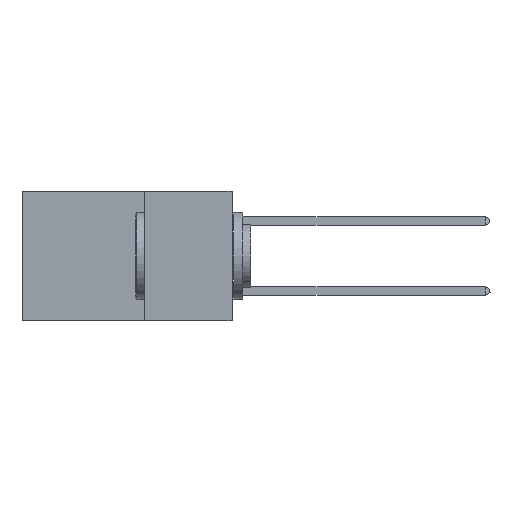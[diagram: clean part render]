
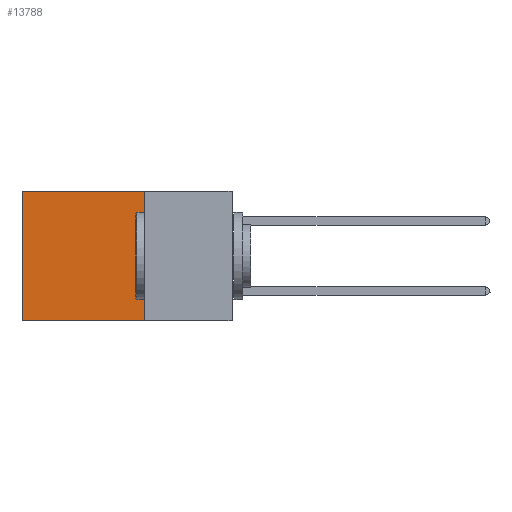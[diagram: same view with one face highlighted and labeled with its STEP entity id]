
A CAD part, left-side view. The second image highlights one B-rep face of the part: STEP entity #13788.
In plain terms, the highlighted planar face has unit normal (-1, 0, 0).
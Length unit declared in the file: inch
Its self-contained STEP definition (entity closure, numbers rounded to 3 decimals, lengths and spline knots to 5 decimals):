
#313 = CARTESIAN_POINT ( 'NONE',  ( 0.2875, 0.25, 0. ) ) ;
#743 = LINE ( 'NONE', #20657, #4376 ) ;
#978 = EDGE_LOOP ( 'NONE', ( #11214, #15715, #9645, #1679 ) ) ;
#1080 = DIRECTION ( 'NONE',  ( 0., 0., -1. ) ) ;
#1398 = CARTESIAN_POINT ( 'NONE',  ( 0.2875, 0.6, -0.37 ) ) ;
#1679 = ORIENTED_EDGE ( 'NONE', *, *, #10819, .T. ) ;
#2163 = DIRECTION ( 'NONE',  ( 0., 1., 0. ) ) ;
#2410 = LINE ( 'NONE', #313, #15535 ) ;
#3400 = DIRECTION ( 'NONE',  ( 1., 0., 0. ) ) ;
#4041 = VERTEX_POINT ( 'NONE', #1398 ) ;
#4376 = VECTOR ( 'NONE', #18829, 39.37008 ) ;
#8440 = DIRECTION ( 'NONE',  ( 0., 0., -1. ) ) ;
#8909 = VECTOR ( 'NONE', #14401, 39.37008 ) ;
#9415 = CARTESIAN_POINT ( 'NONE',  ( 0.2875, 0.25, -0.37 ) ) ;
#9490 = EDGE_CURVE ( 'NONE', #19579, #4041, #10153, .T. ) ;
#9645 = ORIENTED_EDGE ( 'NONE', *, *, #14976, .F. ) ;
#10153 = LINE ( 'NONE', #9415, #8909 ) ;
#10570 = VECTOR ( 'NONE', #1080, 39.37008 ) ;
#10819 = EDGE_CURVE ( 'NONE', #16153, #11920, #2410, .T. ) ;
#11214 = ORIENTED_EDGE ( 'NONE', *, *, #11694, .T. ) ;
#11533 = CARTESIAN_POINT ( 'NONE',  ( 0.2875, 0.25, 0. ) ) ;
#11694 = EDGE_CURVE ( 'NONE', #11920, #4041, #19549, .T. ) ;
#11753 = CARTESIAN_POINT ( 'NONE',  ( 0.2875, 0.6, 0. ) ) ;
#11920 = VERTEX_POINT ( 'NONE', #11753 ) ;
#13788 = ADVANCED_FACE ( 'NONE', ( #21123 ), #16334, .F. ) ;
#14157 = CARTESIAN_POINT ( 'NONE',  ( 0.2875, 0.6, 0. ) ) ;
#14401 = DIRECTION ( 'NONE',  ( 0., 1., 0. ) ) ;
#14976 = EDGE_CURVE ( 'NONE', #16153, #19579, #743, .T. ) ;
#15535 = VECTOR ( 'NONE', #2163, 39.37008 ) ;
#15715 = ORIENTED_EDGE ( 'NONE', *, *, #9490, .F. ) ;
#16153 = VERTEX_POINT ( 'NONE', #11533 ) ;
#16334 = PLANE ( 'NONE',  #21226 ) ;
#16468 = CARTESIAN_POINT ( 'NONE',  ( 0.2875, 0.25, 0. ) ) ;
#18829 = DIRECTION ( 'NONE',  ( 0., 0., -1. ) ) ;
#19115 = CARTESIAN_POINT ( 'NONE',  ( 0.2875, 0.25, -0.37 ) ) ;
#19549 = LINE ( 'NONE', #14157, #10570 ) ;
#19579 = VERTEX_POINT ( 'NONE', #19115 ) ;
#20657 = CARTESIAN_POINT ( 'NONE',  ( 0.2875, 0.25, 0. ) ) ;
#21123 = FACE_OUTER_BOUND ( 'NONE', #978, .T. ) ;
#21226 = AXIS2_PLACEMENT_3D ( 'NONE', #16468, #3400, #8440 ) ;
